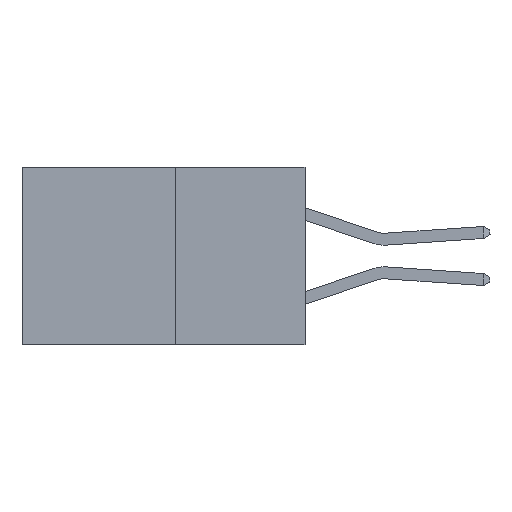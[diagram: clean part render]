
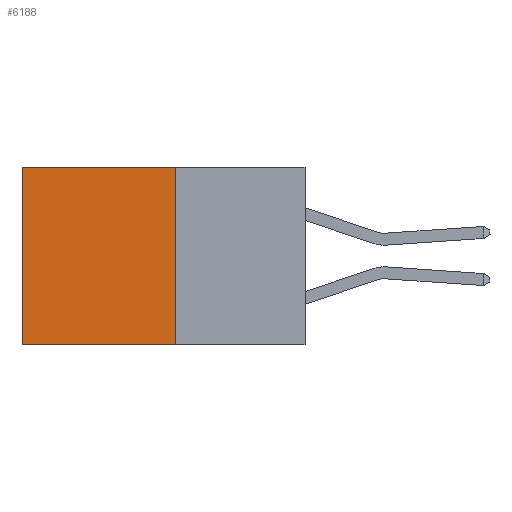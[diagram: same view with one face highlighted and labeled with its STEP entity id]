
A CAD part, left-side view. The second image highlights one B-rep face of the part: STEP entity #6188.
In plain terms, the highlighted planar face has unit normal (-1, 0, 0).
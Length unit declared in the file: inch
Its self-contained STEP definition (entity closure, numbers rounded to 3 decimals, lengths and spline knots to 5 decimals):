
#1452 = VERTEX_POINT ( 'NONE', #11491 ) ;
#1813 = ORIENTED_EDGE ( 'NONE', *, *, #7939, .T. ) ;
#1963 = VECTOR ( 'NONE', #10594, 39.37008 ) ;
#2039 = VECTOR ( 'NONE', #10407, 39.37008 ) ;
#2453 = VERTEX_POINT ( 'NONE', #3385 ) ;
#2859 = EDGE_CURVE ( 'NONE', #1452, #10168, #9189, .T. ) ;
#3280 = ORIENTED_EDGE ( 'NONE', *, *, #2859, .T. ) ;
#3325 = EDGE_LOOP ( 'NONE', ( #1813, #3384, #6538, #3280 ) ) ;
#3384 = ORIENTED_EDGE ( 'NONE', *, *, #4834, .F. ) ;
#3385 = CARTESIAN_POINT ( 'NONE',  ( 0.277, 0.59, -0.37 ) ) ;
#4451 = LINE ( 'NONE', #10813, #1963 ) ;
#4834 = EDGE_CURVE ( 'NONE', #9018, #2453, #11694, .T. ) ;
#5844 = CARTESIAN_POINT ( 'NONE',  ( 0.277, 0.59, 0. ) ) ;
#6168 = CARTESIAN_POINT ( 'NONE',  ( 0.277, 0.27, 0. ) ) ;
#6188 = ADVANCED_FACE ( 'NONE', ( #8961 ), #10760, .F. ) ;
#6538 = ORIENTED_EDGE ( 'NONE', *, *, #9009, .F. ) ;
#6873 = LINE ( 'NONE', #10803, #8893 ) ;
#6930 = VECTOR ( 'NONE', #8004, 39.37008 ) ;
#7939 = EDGE_CURVE ( 'NONE', #10168, #2453, #4451, .T. ) ;
#8004 = DIRECTION ( 'NONE',  ( 0., 1., 0. ) ) ;
#8893 = VECTOR ( 'NONE', #10751, 39.37008 ) ;
#8961 = FACE_OUTER_BOUND ( 'NONE', #3325, .T. ) ;
#9009 = EDGE_CURVE ( 'NONE', #1452, #9018, #6873, .T. ) ;
#9018 = VERTEX_POINT ( 'NONE', #10799 ) ;
#9189 = LINE ( 'NONE', #6168, #6930 ) ;
#10168 = VERTEX_POINT ( 'NONE', #5844 ) ;
#10407 = DIRECTION ( 'NONE',  ( 0., 1., 0. ) ) ;
#10428 = CARTESIAN_POINT ( 'NONE',  ( 0.277, 0.27, -0.37 ) ) ;
#10446 = AXIS2_PLACEMENT_3D ( 'NONE', #10937, #10592, #10476 ) ;
#10476 = DIRECTION ( 'NONE',  ( 0., 0., -1. ) ) ;
#10592 = DIRECTION ( 'NONE',  ( 1., 0., 0. ) ) ;
#10594 = DIRECTION ( 'NONE',  ( 0., 0., -1. ) ) ;
#10751 = DIRECTION ( 'NONE',  ( 0., 0., -1. ) ) ;
#10760 = PLANE ( 'NONE',  #10446 ) ;
#10799 = CARTESIAN_POINT ( 'NONE',  ( 0.277, 0.27, -0.37 ) ) ;
#10803 = CARTESIAN_POINT ( 'NONE',  ( 0.277, 0.27, -0.37 ) ) ;
#10813 = CARTESIAN_POINT ( 'NONE',  ( 0.277, 0.59, -0.37 ) ) ;
#10937 = CARTESIAN_POINT ( 'NONE',  ( 0.277, 0.27, -0.37 ) ) ;
#11491 = CARTESIAN_POINT ( 'NONE',  ( 0.277, 0.27, 0. ) ) ;
#11694 = LINE ( 'NONE', #10428, #2039 ) ;
